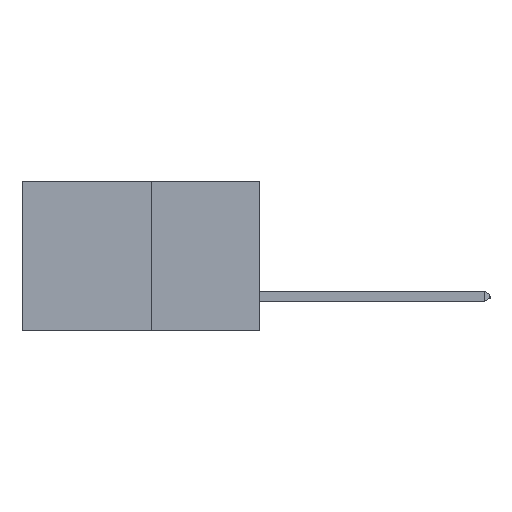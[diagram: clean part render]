
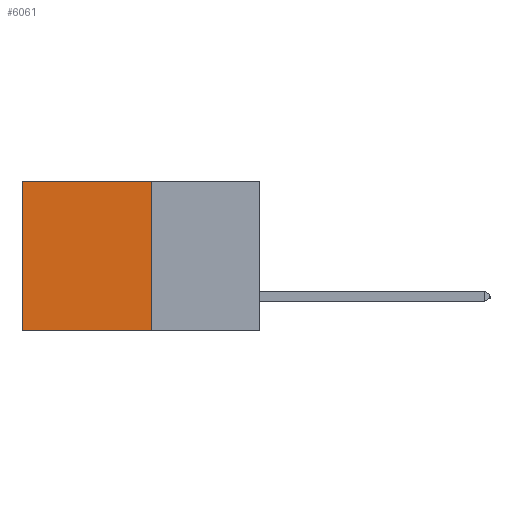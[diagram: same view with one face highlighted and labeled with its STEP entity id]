
A CAD part, left-side view. The second image highlights one B-rep face of the part: STEP entity #6061.
In plain terms, the highlighted planar face has unit normal (-1, 0, 0).
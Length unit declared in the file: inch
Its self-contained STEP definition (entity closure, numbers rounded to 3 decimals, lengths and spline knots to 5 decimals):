
#67 = VERTEX_POINT ( 'NONE', #2022 ) ;
#587 = DIRECTION ( 'NONE',  ( 0., 0., -1. ) ) ;
#835 = EDGE_CURVE ( 'NONE', #8855, #67, #2390, .T. ) ;
#1030 = ORIENTED_EDGE ( 'NONE', *, *, #7244, .F. ) ;
#2022 = CARTESIAN_POINT ( 'NONE',  ( 0.277, 0.27, -0.37 ) ) ;
#2076 = ORIENTED_EDGE ( 'NONE', *, *, #835, .F. ) ;
#2168 = CARTESIAN_POINT ( 'NONE',  ( 0.277, 0.27, 0. ) ) ;
#2390 = LINE ( 'NONE', #8986, #4624 ) ;
#2609 = VECTOR ( 'NONE', #3955, 39.37008 ) ;
#3336 = AXIS2_PLACEMENT_3D ( 'NONE', #8091, #9192, #7127 ) ;
#3664 = ORIENTED_EDGE ( 'NONE', *, *, #8833, .T. ) ;
#3955 = DIRECTION ( 'NONE',  ( 0., 0., -1. ) ) ;
#3986 = CARTESIAN_POINT ( 'NONE',  ( 0.277, 0.59, -0.37 ) ) ;
#4371 = VERTEX_POINT ( 'NONE', #10088 ) ;
#4543 = LINE ( 'NONE', #3986, #2609 ) ;
#4624 = VECTOR ( 'NONE', #587, 39.37008 ) ;
#4733 = EDGE_CURVE ( 'NONE', #8858, #4371, #4543, .T. ) ;
#5013 = DIRECTION ( 'NONE',  ( 0., 1., 0. ) ) ;
#5043 = VECTOR ( 'NONE', #8595, 39.37008 ) ;
#5342 = LINE ( 'NONE', #9384, #5043 ) ;
#5489 = ORIENTED_EDGE ( 'NONE', *, *, #4733, .T. ) ;
#6061 = ADVANCED_FACE ( 'NONE', ( #6115 ), #9093, .F. ) ;
#6115 = FACE_OUTER_BOUND ( 'NONE', #8003, .T. ) ;
#6725 = VECTOR ( 'NONE', #5013, 39.37008 ) ;
#6863 = CARTESIAN_POINT ( 'NONE',  ( 0.277, 0.59, 0. ) ) ;
#7127 = DIRECTION ( 'NONE',  ( 0., 0., -1. ) ) ;
#7244 = EDGE_CURVE ( 'NONE', #67, #4371, #5342, .T. ) ;
#8003 = EDGE_LOOP ( 'NONE', ( #5489, #1030, #2076, #3664 ) ) ;
#8091 = CARTESIAN_POINT ( 'NONE',  ( 0.277, 0.27, -0.37 ) ) ;
#8520 = CARTESIAN_POINT ( 'NONE',  ( 0.277, 0.27, 0. ) ) ;
#8595 = DIRECTION ( 'NONE',  ( 0., 1., 0. ) ) ;
#8833 = EDGE_CURVE ( 'NONE', #8855, #8858, #9018, .T. ) ;
#8855 = VERTEX_POINT ( 'NONE', #2168 ) ;
#8858 = VERTEX_POINT ( 'NONE', #6863 ) ;
#8986 = CARTESIAN_POINT ( 'NONE',  ( 0.277, 0.27, -0.37 ) ) ;
#9018 = LINE ( 'NONE', #8520, #6725 ) ;
#9093 = PLANE ( 'NONE',  #3336 ) ;
#9192 = DIRECTION ( 'NONE',  ( 1., 0., 0. ) ) ;
#9384 = CARTESIAN_POINT ( 'NONE',  ( 0.277, 0.27, -0.37 ) ) ;
#10088 = CARTESIAN_POINT ( 'NONE',  ( 0.277, 0.59, -0.37 ) ) ;
